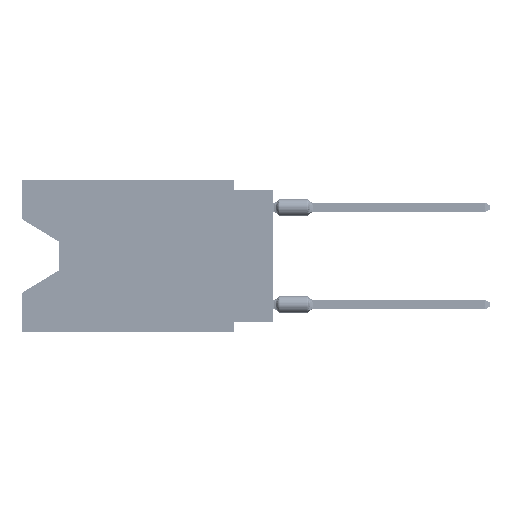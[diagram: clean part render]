
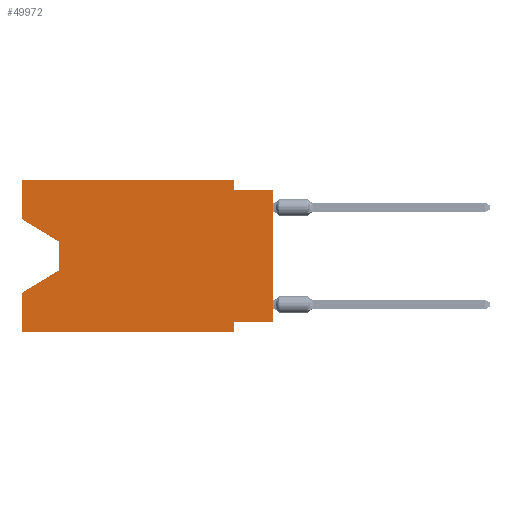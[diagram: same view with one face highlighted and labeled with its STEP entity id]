
A CAD part, left-side view. The second image highlights one B-rep face of the part: STEP entity #49972.
In plain terms, the highlighted planar face has unit normal (-1, 0, 0).
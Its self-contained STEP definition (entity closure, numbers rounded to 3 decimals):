
#191 = ORIENTED_EDGE ( 'NONE', *, *, #71741, .T. ) ;
#3424 = VERTEX_POINT ( 'NONE', #47573 ) ;
#3760 = CARTESIAN_POINT ( 'NONE',  ( 0., 0., -0.635 ) ) ;
#4247 = LINE ( 'NONE', #17690, #30729 ) ;
#9081 = ORIENTED_EDGE ( 'NONE', *, *, #23494, .T. ) ;
#9533 = LINE ( 'NONE', #11195, #25652 ) ;
#10214 = CARTESIAN_POINT ( 'NONE',  ( 0., 13.97, -4.013 ) ) ;
#10621 = ORIENTED_EDGE ( 'NONE', *, *, #21187, .T. ) ;
#10639 = LINE ( 'NONE', #61888, #24899 ) ;
#10962 = CARTESIAN_POINT ( 'NONE',  ( 0., 2.54, 0. ) ) ;
#11195 = CARTESIAN_POINT ( 'NONE',  ( 0., 2.54, -9.906 ) ) ;
#11738 = LINE ( 'NONE', #49509, #34531 ) ;
#14095 = ORIENTED_EDGE ( 'NONE', *, *, #20540, .T. ) ;
#17049 = VECTOR ( 'NONE', #73523, 1000. ) ;
#17690 = CARTESIAN_POINT ( 'NONE',  ( 0., 0., -9.271 ) ) ;
#18730 = VECTOR ( 'NONE', #26785, 1000. ) ;
#18741 = DIRECTION ( 'NONE',  ( 0., 0., 1. ) ) ;
#18745 = CARTESIAN_POINT ( 'NONE',  ( 0., 16.383, -2.546 ) ) ;
#18857 = ORIENTED_EDGE ( 'NONE', *, *, #79178, .F. ) ;
#19328 = DIRECTION ( 'NONE',  ( 0., 0., 1. ) ) ;
#20540 = EDGE_CURVE ( 'NONE', #51076, #50689, #35677, .T. ) ;
#21086 = VECTOR ( 'NONE', #18741, 1000. ) ;
#21187 = EDGE_CURVE ( 'NONE', #3424, #37572, #31337, .T. ) ;
#23304 = CARTESIAN_POINT ( 'NONE',  ( 0., 16.383, 0. ) ) ;
#23494 = EDGE_CURVE ( 'NONE', #34563, #63506, #58253, .T. ) ;
#23496 = CARTESIAN_POINT ( 'NONE',  ( 0., 16.383, -9.906 ) ) ;
#24202 = DIRECTION ( 'NONE',  ( 0., 0.855, -0.519 ) ) ;
#24899 = VECTOR ( 'NONE', #55575, 1000. ) ;
#24915 = CARTESIAN_POINT ( 'NONE',  ( 0., 16.383, 0. ) ) ;
#25414 = CARTESIAN_POINT ( 'NONE',  ( 0., 13.97, -5.893 ) ) ;
#25652 = VECTOR ( 'NONE', #48164, 1000. ) ;
#26785 = DIRECTION ( 'NONE',  ( 0., -1., 0. ) ) ;
#27429 = EDGE_CURVE ( 'NONE', #82973, #31794, #11738, .T. ) ;
#28231 = VECTOR ( 'NONE', #43937, 1000. ) ;
#30407 = EDGE_CURVE ( 'NONE', #54524, #82973, #59957, .T. ) ;
#30729 = VECTOR ( 'NONE', #49187, 1000. ) ;
#30908 = VECTOR ( 'NONE', #19328, 1000. ) ;
#31337 = LINE ( 'NONE', #38469, #21086 ) ;
#31690 = VERTEX_POINT ( 'NONE', #48159 ) ;
#31728 = CARTESIAN_POINT ( 'NONE',  ( 0., 2.54, -9.906 ) ) ;
#31794 = VERTEX_POINT ( 'NONE', #36851 ) ;
#32708 = VECTOR ( 'NONE', #24202, 1000. ) ;
#33777 = ORIENTED_EDGE ( 'NONE', *, *, #27429, .F. ) ;
#34181 = EDGE_LOOP ( 'NONE', ( #43633, #9081, #191, #34411, #14095, #79489, #56283, #10621, #56054, #33777, #35435, #18857 ) ) ;
#34411 = ORIENTED_EDGE ( 'NONE', *, *, #39231, .F. ) ;
#34531 = VECTOR ( 'NONE', #55438, 1000. ) ;
#34563 = VERTEX_POINT ( 'NONE', #10214 ) ;
#35435 = ORIENTED_EDGE ( 'NONE', *, *, #30407, .F. ) ;
#35677 = LINE ( 'NONE', #23496, #74634 ) ;
#36851 = CARTESIAN_POINT ( 'NONE',  ( 0., 2.54, -0.635 ) ) ;
#37572 = VERTEX_POINT ( 'NONE', #45133 ) ;
#38469 = CARTESIAN_POINT ( 'NONE',  ( 0., 0., 0. ) ) ;
#39231 = EDGE_CURVE ( 'NONE', #51076, #61465, #10639, .T. ) ;
#39339 = CARTESIAN_POINT ( 'NONE',  ( 0., 13.97, -4.013 ) ) ;
#42231 = EDGE_CURVE ( 'NONE', #3424, #69593, #4247, .T. ) ;
#43633 = ORIENTED_EDGE ( 'NONE', *, *, #59231, .T. ) ;
#43918 = LINE ( 'NONE', #49794, #32708 ) ;
#43937 = DIRECTION ( 'NONE',  ( 0., -0.855, -0.519 ) ) ;
#44577 = EDGE_CURVE ( 'NONE', #69593, #50689, #9533, .T. ) ;
#45133 = CARTESIAN_POINT ( 'NONE',  ( 0., 0., -0.635 ) ) ;
#46080 = CARTESIAN_POINT ( 'NONE',  ( 0., 16.383, 0. ) ) ;
#46658 = CARTESIAN_POINT ( 'NONE',  ( 0., 16.383, -7.36 ) ) ;
#47573 = CARTESIAN_POINT ( 'NONE',  ( 0., 0., -9.271 ) ) ;
#48159 = CARTESIAN_POINT ( 'NONE',  ( 0., 16.383, -2.546 ) ) ;
#48164 = DIRECTION ( 'NONE',  ( 0., 0., -1. ) ) ;
#49096 = DIRECTION ( 'NONE',  ( 0., -1., 0. ) ) ;
#49187 = DIRECTION ( 'NONE',  ( 0., 1., 0. ) ) ;
#49509 = CARTESIAN_POINT ( 'NONE',  ( 0., 2.54, 0. ) ) ;
#49794 = CARTESIAN_POINT ( 'NONE',  ( 0., 13.97, -5.893 ) ) ;
#49972 = ADVANCED_FACE ( 'NONE', ( #56827 ), #82461, .F. ) ;
#50494 = DIRECTION ( 'NONE',  ( 1., 0., 0. ) ) ;
#50689 = VERTEX_POINT ( 'NONE', #31728 ) ;
#50807 = LINE ( 'NONE', #56299, #30908 ) ;
#51076 = VERTEX_POINT ( 'NONE', #69437 ) ;
#53336 = EDGE_CURVE ( 'NONE', #31794, #37572, #61316, .T. ) ;
#54524 = VERTEX_POINT ( 'NONE', #23304 ) ;
#55438 = DIRECTION ( 'NONE',  ( 0., 0., -1. ) ) ;
#55575 = DIRECTION ( 'NONE',  ( 0., 0., 1. ) ) ;
#56054 = ORIENTED_EDGE ( 'NONE', *, *, #53336, .F. ) ;
#56283 = ORIENTED_EDGE ( 'NONE', *, *, #42231, .F. ) ;
#56299 = CARTESIAN_POINT ( 'NONE',  ( 0., 16.383, 0. ) ) ;
#56827 = FACE_OUTER_BOUND ( 'NONE', #34181, .T. ) ;
#57805 = LINE ( 'NONE', #18745, #28231 ) ;
#58247 = AXIS2_PLACEMENT_3D ( 'NONE', #24915, #50494, #76164 ) ;
#58253 = LINE ( 'NONE', #39339, #61535 ) ;
#59231 = EDGE_CURVE ( 'NONE', #31690, #34563, #57805, .T. ) ;
#59957 = LINE ( 'NONE', #46080, #18730 ) ;
#61316 = LINE ( 'NONE', #3760, #17049 ) ;
#61465 = VERTEX_POINT ( 'NONE', #46658 ) ;
#61535 = VECTOR ( 'NONE', #64975, 1000. ) ;
#61888 = CARTESIAN_POINT ( 'NONE',  ( 0., 16.383, 0. ) ) ;
#63506 = VERTEX_POINT ( 'NONE', #25414 ) ;
#64975 = DIRECTION ( 'NONE',  ( 0., 0., -1. ) ) ;
#69437 = CARTESIAN_POINT ( 'NONE',  ( 0., 16.383, -9.906 ) ) ;
#69593 = VERTEX_POINT ( 'NONE', #75502 ) ;
#71741 = EDGE_CURVE ( 'NONE', #63506, #61465, #43918, .T. ) ;
#73523 = DIRECTION ( 'NONE',  ( 0., -1., 0. ) ) ;
#74634 = VECTOR ( 'NONE', #49096, 1000. ) ;
#75502 = CARTESIAN_POINT ( 'NONE',  ( 0., 2.54, -9.271 ) ) ;
#76164 = DIRECTION ( 'NONE',  ( 0., 0., -1. ) ) ;
#79178 = EDGE_CURVE ( 'NONE', #31690, #54524, #50807, .T. ) ;
#79489 = ORIENTED_EDGE ( 'NONE', *, *, #44577, .F. ) ;
#82461 = PLANE ( 'NONE',  #58247 ) ;
#82973 = VERTEX_POINT ( 'NONE', #10962 ) ;
